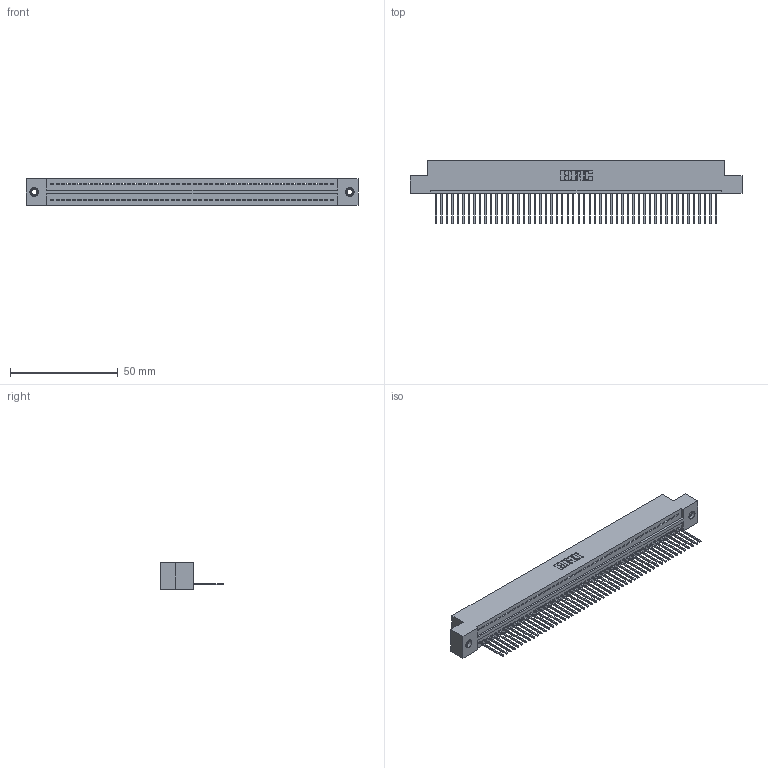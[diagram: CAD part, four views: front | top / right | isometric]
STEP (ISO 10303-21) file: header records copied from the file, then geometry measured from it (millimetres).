
FILE_DESCRIPTION (( 'STEP AP203' ), '1' );
FILE_NAME ('325-052-540-107.STEP', '2020-02-25T00:29:11', ( '' ), ( '' ), 'SwSTEP 2.0', 'SolidWorks 2016', '' );
FILE_SCHEMA (( 'CONFIG_CONTROL_DESIGN' ));
Length unit declared in the file: inch
Products named in the file (4): 325-292-001_325-293-140; 345-250-001_345-250-005-103; 325 Part_TI; 325-052-540-107
Assembly tree (55 placements, depth 2):
  325-052-540-107
    325 Part_TI
    325-292-001_325-293-140  x52
    345-250-001_345-250-005-103  x2
Bounding box: 153.8 x 29.46 x 12.45 mm (x, y, z)
Volume: 19660.3 mm3; surface area: 22196.6 mm2
Topology: 55 solids, 55 shells, 3190 faces, 9599 edges, 6322 vertices
Faces by surface type: plane 2286, cylinder 888, cone 12, torus 4
Entity records: 31700 total; most frequent: CARTESIAN_POINT 5449, ORIENTED_EDGE 5430, DIRECTION 4609, EDGE_CURVE 2715, VECTOR 2567, LINE 2567, VERTEX_POINT 1804, AXIS2_PLACEMENT_3D 1021
